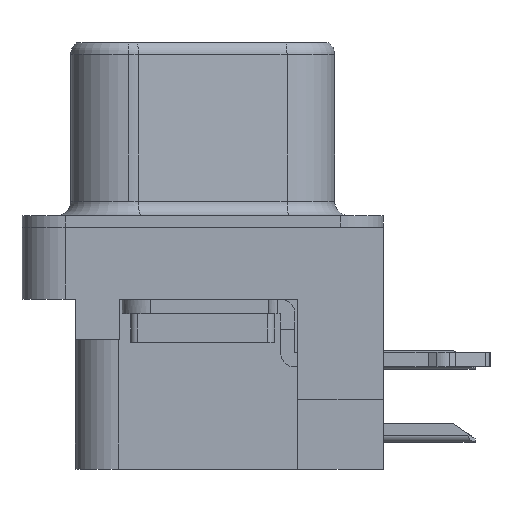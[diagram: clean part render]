
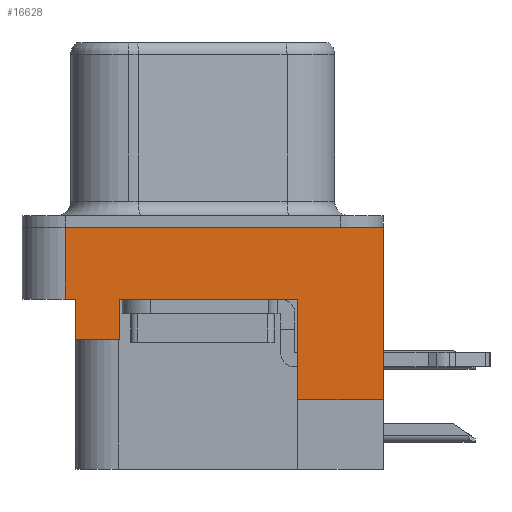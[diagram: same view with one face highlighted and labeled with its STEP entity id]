
A CAD part, left-side view. The second image highlights one B-rep face of the part: STEP entity #16628.
In plain terms, the highlighted planar face has unit normal (-1, 0, 0).
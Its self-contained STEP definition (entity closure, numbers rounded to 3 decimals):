
#130 = EDGE_CURVE ( 'NONE', #10856, #1691, #16317, .T. ) ;
#203 = LINE ( 'NONE', #14080, #14923 ) ;
#484 = DIRECTION ( 'NONE',  ( 0., -1., 0. ) ) ;
#1227 = VECTOR ( 'NONE', #14505, 1000. ) ;
#1337 = FACE_OUTER_BOUND ( 'NONE', #12209, .T. ) ;
#1350 = LINE ( 'NONE', #12166, #16580 ) ;
#1678 = LINE ( 'NONE', #3592, #1227 ) ;
#1691 = VERTEX_POINT ( 'NONE', #2139 ) ;
#1756 = EDGE_CURVE ( 'NONE', #10877, #11170, #1678, .T. ) ;
#2139 = CARTESIAN_POINT ( 'NONE',  ( -2.935, 2.895, -2.5 ) ) ;
#2325 = VERTEX_POINT ( 'NONE', #6100 ) ;
#2468 = ORIENTED_EDGE ( 'NONE', *, *, #8016, .F. ) ;
#2572 = CARTESIAN_POINT ( 'NONE',  ( -2.935, -6.275, -2.5 ) ) ;
#2613 = DIRECTION ( 'NONE',  ( 0., 1., 0. ) ) ;
#2836 = VECTOR ( 'NONE', #16370, 1000. ) ;
#2843 = ORIENTED_EDGE ( 'NONE', *, *, #13160, .T. ) ;
#2866 = DIRECTION ( 'NONE',  ( 0., 0., 1. ) ) ;
#3011 = CARTESIAN_POINT ( 'NONE',  ( -2.935, -6.275, 0. ) ) ;
#3309 = LINE ( 'NONE', #11855, #2836 ) ;
#3538 = CARTESIAN_POINT ( 'NONE',  ( -2.935, 4.425, -3.9 ) ) ;
#3592 = CARTESIAN_POINT ( 'NONE',  ( -2.935, -6.495, -6. ) ) ;
#3739 = VERTEX_POINT ( 'NONE', #8532 ) ;
#3906 = LINE ( 'NONE', #18833, #15649 ) ;
#4465 = CARTESIAN_POINT ( 'NONE',  ( -2.935, -6.275, -6. ) ) ;
#4501 = DIRECTION ( 'NONE',  ( 0., -1., 0. ) ) ;
#4716 = VECTOR ( 'NONE', #17860, 1000. ) ;
#5122 = ORIENTED_EDGE ( 'NONE', *, *, #13535, .T. ) ;
#5158 = ORIENTED_EDGE ( 'NONE', *, *, #8622, .T. ) ;
#5167 = LINE ( 'NONE', #17580, #15043 ) ;
#6100 = CARTESIAN_POINT ( 'NONE',  ( -2.935, 4.425, -2.5 ) ) ;
#8016 = EDGE_CURVE ( 'NONE', #11649, #2325, #16495, .T. ) ;
#8408 = VECTOR ( 'NONE', #15737, 1000. ) ;
#8434 = VECTOR ( 'NONE', #4501, 1000. ) ;
#8446 = DIRECTION ( 'NONE',  ( -1., 0., 0. ) ) ;
#8532 = CARTESIAN_POINT ( 'NONE',  ( -2.935, -6.275, 0. ) ) ;
#8622 = EDGE_CURVE ( 'NONE', #10877, #3739, #5167, .T. ) ;
#8715 = DIRECTION ( 'NONE',  ( 0., -1., 0. ) ) ;
#8897 = LINE ( 'NONE', #3011, #8434 ) ;
#9961 = EDGE_CURVE ( 'NONE', #11170, #17429, #3309, .T. ) ;
#10024 = ORIENTED_EDGE ( 'NONE', *, *, #9961, .F. ) ;
#10364 = ORIENTED_EDGE ( 'NONE', *, *, #12783, .F. ) ;
#10491 = VECTOR ( 'NONE', #8715, 1000. ) ;
#10856 = VERTEX_POINT ( 'NONE', #14661 ) ;
#10877 = VERTEX_POINT ( 'NONE', #4465 ) ;
#11170 = VERTEX_POINT ( 'NONE', #13869 ) ;
#11196 = DIRECTION ( 'NONE',  ( 0., 0., 1. ) ) ;
#11428 = AXIS2_PLACEMENT_3D ( 'NONE', #2572, #8446, #18857 ) ;
#11649 = VERTEX_POINT ( 'NONE', #3538 ) ;
#11663 = ORIENTED_EDGE ( 'NONE', *, *, #130, .T. ) ;
#11855 = CARTESIAN_POINT ( 'NONE',  ( -2.935, -3.295, -8.4 ) ) ;
#12166 = CARTESIAN_POINT ( 'NONE',  ( -2.935, -6.275, -2.5 ) ) ;
#12209 = EDGE_LOOP ( 'NONE', ( #13860, #5158, #14901, #15224, #2843, #2468, #10364, #11663, #5122, #10024 ) ) ;
#12783 = EDGE_CURVE ( 'NONE', #10856, #11649, #3906, .T. ) ;
#12903 = CARTESIAN_POINT ( 'NONE',  ( -2.935, 2.895, -3.9 ) ) ;
#12951 = EDGE_CURVE ( 'NONE', #16511, #3739, #8897, .T. ) ;
#13160 = EDGE_CURVE ( 'NONE', #13628, #2325, #1350, .T. ) ;
#13364 = CARTESIAN_POINT ( 'NONE',  ( -2.935, 4.775, -2.5 ) ) ;
#13535 = EDGE_CURVE ( 'NONE', #1691, #17429, #17946, .T. ) ;
#13628 = VERTEX_POINT ( 'NONE', #13364 ) ;
#13860 = ORIENTED_EDGE ( 'NONE', *, *, #1756, .F. ) ;
#13869 = CARTESIAN_POINT ( 'NONE',  ( -2.935, -3.295, -6. ) ) ;
#14064 = CARTESIAN_POINT ( 'NONE',  ( -2.935, 4.775, 0. ) ) ;
#14080 = CARTESIAN_POINT ( 'NONE',  ( -2.935, 4.775, -2.5 ) ) ;
#14332 = PLANE ( 'NONE',  #11428 ) ;
#14505 = DIRECTION ( 'NONE',  ( 0., 1., 0. ) ) ;
#14661 = CARTESIAN_POINT ( 'NONE',  ( -2.935, 2.895, -3.9 ) ) ;
#14764 = CARTESIAN_POINT ( 'NONE',  ( -2.935, -3.295, -2.5 ) ) ;
#14901 = ORIENTED_EDGE ( 'NONE', *, *, #12951, .F. ) ;
#14923 = VECTOR ( 'NONE', #11196, 1000. ) ;
#15043 = VECTOR ( 'NONE', #2866, 1000. ) ;
#15224 = ORIENTED_EDGE ( 'NONE', *, *, #15955, .F. ) ;
#15649 = VECTOR ( 'NONE', #2613, 1000. ) ;
#15737 = DIRECTION ( 'NONE',  ( 0., 0., 1. ) ) ;
#15955 = EDGE_CURVE ( 'NONE', #13628, #16511, #203, .T. ) ;
#16133 = CARTESIAN_POINT ( 'NONE',  ( -2.935, -6.275, -2.5 ) ) ;
#16297 = CARTESIAN_POINT ( 'NONE',  ( -2.935, 4.425, -3.9 ) ) ;
#16317 = LINE ( 'NONE', #12903, #8408 ) ;
#16370 = DIRECTION ( 'NONE',  ( 0., 0., 1. ) ) ;
#16495 = LINE ( 'NONE', #16297, #4716 ) ;
#16511 = VERTEX_POINT ( 'NONE', #14064 ) ;
#16580 = VECTOR ( 'NONE', #484, 1000. ) ;
#16628 = ADVANCED_FACE ( 'NONE', ( #1337 ), #14332, .T. ) ;
#17429 = VERTEX_POINT ( 'NONE', #14764 ) ;
#17580 = CARTESIAN_POINT ( 'NONE',  ( -2.935, -6.275, -2.5 ) ) ;
#17860 = DIRECTION ( 'NONE',  ( 0., 0., 1. ) ) ;
#17946 = LINE ( 'NONE', #16133, #10491 ) ;
#18833 = CARTESIAN_POINT ( 'NONE',  ( -2.935, 4.425, -3.9 ) ) ;
#18857 = DIRECTION ( 'NONE',  ( 0., 0., 1. ) ) ;
